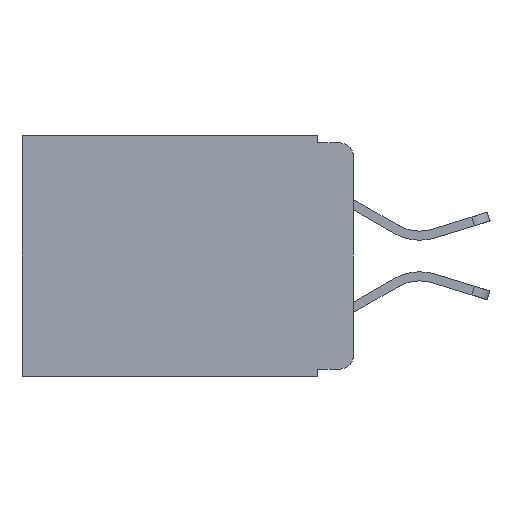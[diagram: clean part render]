
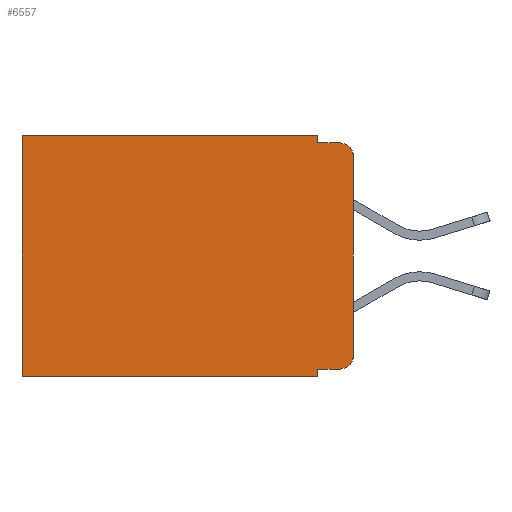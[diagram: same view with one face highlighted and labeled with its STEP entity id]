
A CAD part, left-side view. The second image highlights one B-rep face of the part: STEP entity #6557.
In plain terms, the highlighted planar face has unit normal (-1, 0, 0).
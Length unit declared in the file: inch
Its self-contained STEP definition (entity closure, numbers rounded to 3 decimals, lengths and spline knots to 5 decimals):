
#197 = LINE ( 'NONE', #7054, #18569 ) ;
#878 = DIRECTION ( 'NONE',  ( 0., -1., 0. ) ) ;
#1225 = CIRCLE ( 'NONE', #16488, 0.02 ) ;
#1617 = VERTEX_POINT ( 'NONE', #2701 ) ;
#1626 = ORIENTED_EDGE ( 'NONE', *, *, #6507, .F. ) ;
#2586 = VECTOR ( 'NONE', #9533, 39.37008 ) ;
#2607 = VECTOR ( 'NONE', #878, 39.37008 ) ;
#2701 = CARTESIAN_POINT ( 'NONE',  ( 0.298, 0.051, -0.343 ) ) ;
#2711 = ORIENTED_EDGE ( 'NONE', *, *, #6838, .T. ) ;
#2871 = VECTOR ( 'NONE', #10482, 39.37008 ) ;
#2909 = ORIENTED_EDGE ( 'NONE', *, *, #6566, .T. ) ;
#3081 = CARTESIAN_POINT ( 'NONE',  ( 0.298, 0.02, -0.01 ) ) ;
#3169 = VECTOR ( 'NONE', #4874, 39.37008 ) ;
#3236 = ORIENTED_EDGE ( 'NONE', *, *, #5823, .F. ) ;
#3674 = LINE ( 'NONE', #14661, #3169 ) ;
#3891 = EDGE_CURVE ( 'NONE', #1617, #6128, #5582, .T. ) ;
#4778 = CARTESIAN_POINT ( 'NONE',  ( 0.298, 0.473, -0.343 ) ) ;
#4874 = DIRECTION ( 'NONE',  ( 0., 0., -1. ) ) ;
#4935 = EDGE_CURVE ( 'NONE', #10261, #6465, #15944, .T. ) ;
#5582 = LINE ( 'NONE', #17156, #16219 ) ;
#5641 = FACE_OUTER_BOUND ( 'NONE', #14874, .T. ) ;
#5643 = ORIENTED_EDGE ( 'NONE', *, *, #3891, .F. ) ;
#5690 = VERTEX_POINT ( 'NONE', #14265 ) ;
#5823 = EDGE_CURVE ( 'NONE', #13257, #14519, #3674, .T. ) ;
#6128 = VERTEX_POINT ( 'NONE', #4778 ) ;
#6314 = EDGE_CURVE ( 'NONE', #6465, #6128, #197, .T. ) ;
#6398 = PLANE ( 'NONE',  #12961 ) ;
#6402 = EDGE_CURVE ( 'NONE', #14288, #18488, #10578, .T. ) ;
#6432 = EDGE_CURVE ( 'NONE', #10261, #5690, #9302, .T. ) ;
#6465 = VERTEX_POINT ( 'NONE', #10302 ) ;
#6507 = EDGE_CURVE ( 'NONE', #14288, #1617, #10774, .T. ) ;
#6513 = CARTESIAN_POINT ( 'NONE',  ( 0.298, 0., -0.03 ) ) ;
#6557 = ADVANCED_FACE ( 'NONE', ( #5641 ), #6398, .F. ) ;
#6566 = EDGE_CURVE ( 'NONE', #18488, #14519, #12685, .T. ) ;
#6654 = EDGE_CURVE ( 'NONE', #5690, #8812, #10973, .T. ) ;
#6838 = EDGE_CURVE ( 'NONE', #13257, #8812, #1225, .T. ) ;
#7042 = CARTESIAN_POINT ( 'NONE',  ( 0.298, 0., -0.313 ) ) ;
#7054 = CARTESIAN_POINT ( 'NONE',  ( 0.298, 0.473, 0. ) ) ;
#7400 = DIRECTION ( 'NONE',  ( -1., 0., 0. ) ) ;
#7773 = CARTESIAN_POINT ( 'NONE',  ( 0.298, 0.051, 0. ) ) ;
#7840 = CARTESIAN_POINT ( 'NONE',  ( 0.298, 0., 0. ) ) ;
#7906 = DIRECTION ( 'NONE',  ( 0., 0., -1. ) ) ;
#8206 = CARTESIAN_POINT ( 'NONE',  ( 0.298, 0.051, -0.01 ) ) ;
#8812 = VERTEX_POINT ( 'NONE', #3081 ) ;
#8873 = VECTOR ( 'NONE', #12923, 39.37008 ) ;
#9112 = CARTESIAN_POINT ( 'NONE',  ( 0.298, 0.051, 0. ) ) ;
#9302 = LINE ( 'NONE', #14275, #8873 ) ;
#9349 = CARTESIAN_POINT ( 'NONE',  ( 0.298, 0.02, -0.313 ) ) ;
#9533 = DIRECTION ( 'NONE',  ( 0., -1., 0. ) ) ;
#9664 = DIRECTION ( 'NONE',  ( 0., 1., 0. ) ) ;
#10025 = ORIENTED_EDGE ( 'NONE', *, *, #6402, .T. ) ;
#10137 = CARTESIAN_POINT ( 'NONE',  ( 0.298, 0.051, -0.333 ) ) ;
#10261 = VERTEX_POINT ( 'NONE', #7773 ) ;
#10302 = CARTESIAN_POINT ( 'NONE',  ( 0.298, 0.473, 0. ) ) ;
#10337 = DIRECTION ( 'NONE',  ( 0., 1., 0. ) ) ;
#10482 = DIRECTION ( 'NONE',  ( 0., 0., -1. ) ) ;
#10578 = LINE ( 'NONE', #10137, #2607 ) ;
#10711 = DIRECTION ( 'NONE',  ( 0., 0., -1. ) ) ;
#10774 = LINE ( 'NONE', #9112, #2871 ) ;
#10973 = LINE ( 'NONE', #8206, #2586 ) ;
#11872 = ORIENTED_EDGE ( 'NONE', *, *, #6432, .F. ) ;
#11909 = CARTESIAN_POINT ( 'NONE',  ( 0.298, 0.02, -0.333 ) ) ;
#12188 = CARTESIAN_POINT ( 'NONE',  ( 0.298, 0.051, -0.333 ) ) ;
#12350 = VECTOR ( 'NONE', #10337, 39.37008 ) ;
#12435 = ORIENTED_EDGE ( 'NONE', *, *, #6654, .F. ) ;
#12660 = ORIENTED_EDGE ( 'NONE', *, *, #4935, .T. ) ;
#12685 = CIRCLE ( 'NONE', #13875, 0.02 ) ;
#12923 = DIRECTION ( 'NONE',  ( 0., 0., -1. ) ) ;
#12961 = AXIS2_PLACEMENT_3D ( 'NONE', #7840, #16026, #7906 ) ;
#13257 = VERTEX_POINT ( 'NONE', #6513 ) ;
#13875 = AXIS2_PLACEMENT_3D ( 'NONE', #9349, #18754, #10711 ) ;
#14265 = CARTESIAN_POINT ( 'NONE',  ( 0.298, 0.051, -0.01 ) ) ;
#14275 = CARTESIAN_POINT ( 'NONE',  ( 0.298, 0.051, 0. ) ) ;
#14288 = VERTEX_POINT ( 'NONE', #12188 ) ;
#14519 = VERTEX_POINT ( 'NONE', #7042 ) ;
#14661 = CARTESIAN_POINT ( 'NONE',  ( 0.298, 0., 0. ) ) ;
#14874 = EDGE_LOOP ( 'NONE', ( #3236, #2711, #12435, #11872, #12660, #15186, #5643, #1626, #10025, #2909 ) ) ;
#15186 = ORIENTED_EDGE ( 'NONE', *, *, #6314, .T. ) ;
#15257 = DIRECTION ( 'NONE',  ( 0., 0., -1. ) ) ;
#15532 = CARTESIAN_POINT ( 'NONE',  ( 0.298, 0.02, -0.03 ) ) ;
#15698 = CARTESIAN_POINT ( 'NONE',  ( 0.298, 0., 0. ) ) ;
#15944 = LINE ( 'NONE', #15698, #12350 ) ;
#16026 = DIRECTION ( 'NONE',  ( 1., 0., 0. ) ) ;
#16219 = VECTOR ( 'NONE', #9664, 39.37008 ) ;
#16488 = AXIS2_PLACEMENT_3D ( 'NONE', #15532, #7400, #16920 ) ;
#16920 = DIRECTION ( 'NONE',  ( 0., 0., -1. ) ) ;
#17156 = CARTESIAN_POINT ( 'NONE',  ( 0.298, 0., -0.343 ) ) ;
#18488 = VERTEX_POINT ( 'NONE', #11909 ) ;
#18569 = VECTOR ( 'NONE', #15257, 39.37008 ) ;
#18754 = DIRECTION ( 'NONE',  ( -1., 0., 0. ) ) ;
